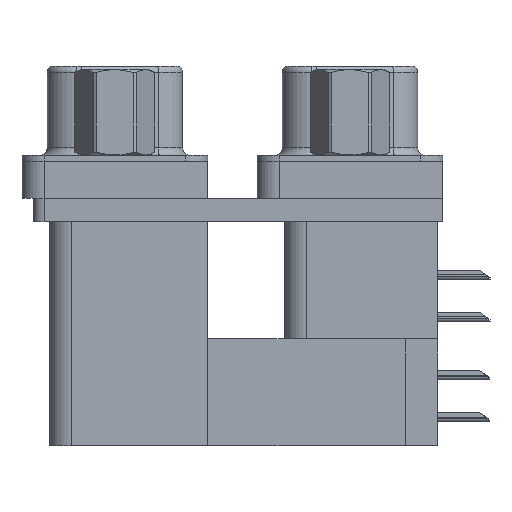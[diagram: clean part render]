
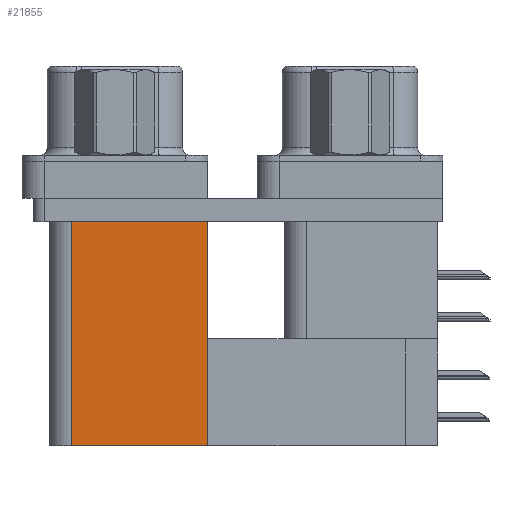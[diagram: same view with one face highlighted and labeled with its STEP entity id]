
A CAD part, left-side view. The second image highlights one B-rep face of the part: STEP entity #21855.
In plain terms, the highlighted planar face has unit normal (-1, 0, 0).
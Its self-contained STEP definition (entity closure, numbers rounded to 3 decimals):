
#1207 = PLANE ( 'NONE',  #14484 ) ;
#2067 = VERTEX_POINT ( 'NONE', #24775 ) ;
#2484 = VECTOR ( 'NONE', #4915, 1000. ) ;
#2681 = LINE ( 'NONE', #6771, #27761 ) ;
#4915 = DIRECTION ( 'NONE',  ( 0., 0., 1. ) ) ;
#5974 = VERTEX_POINT ( 'NONE', #7982 ) ;
#6165 = DIRECTION ( 'NONE',  ( 0., 0., 1. ) ) ;
#6771 = CARTESIAN_POINT ( 'NONE',  ( 3.7, 9.6, -19.2 ) ) ;
#7982 = CARTESIAN_POINT ( 'NONE',  ( 3.7, 9.6, -19.2 ) ) ;
#8665 = EDGE_CURVE ( 'NONE', #5974, #22039, #2681, .T. ) ;
#9884 = ORIENTED_EDGE ( 'NONE', *, *, #22819, .F. ) ;
#11655 = CARTESIAN_POINT ( 'NONE',  ( 3.7, 9.6, -19.2 ) ) ;
#13411 = LINE ( 'NONE', #20430, #40462 ) ;
#14484 = AXIS2_PLACEMENT_3D ( 'NONE', #11655, #32255, #31804 ) ;
#20430 = CARTESIAN_POINT ( 'NONE',  ( 3.7, 18.8, -19.2 ) ) ;
#20454 = CARTESIAN_POINT ( 'NONE',  ( 3.7, 18.8, -19.2 ) ) ;
#20587 = DIRECTION ( 'NONE',  ( 0., 1., 0. ) ) ;
#20968 = ORIENTED_EDGE ( 'NONE', *, *, #8665, .F. ) ;
#21855 = ADVANCED_FACE ( 'NONE', ( #35194 ), #1207, .F. ) ;
#22039 = VERTEX_POINT ( 'NONE', #20454 ) ;
#22819 = EDGE_CURVE ( 'NONE', #22039, #27255, #13411, .T. ) ;
#23968 = ORIENTED_EDGE ( 'NONE', *, *, #31634, .T. ) ;
#24775 = CARTESIAN_POINT ( 'NONE',  ( 3.7, 9.6, -2.5 ) ) ;
#26036 = DIRECTION ( 'NONE',  ( 0., 1., 0. ) ) ;
#26537 = CARTESIAN_POINT ( 'NONE',  ( 3.7, 18.8, -2.5 ) ) ;
#27255 = VERTEX_POINT ( 'NONE', #26537 ) ;
#27761 = VECTOR ( 'NONE', #20587, 1000. ) ;
#29147 = CARTESIAN_POINT ( 'NONE',  ( 3.7, 9.6, -19.2 ) ) ;
#31634 = EDGE_CURVE ( 'NONE', #2067, #27255, #36011, .T. ) ;
#31804 = DIRECTION ( 'NONE',  ( 0., 0., -1. ) ) ;
#32255 = DIRECTION ( 'NONE',  ( 1., 0., 0. ) ) ;
#32833 = CARTESIAN_POINT ( 'NONE',  ( 3.7, 9.6, -2.5 ) ) ;
#35194 = FACE_OUTER_BOUND ( 'NONE', #42204, .T. ) ;
#36011 = LINE ( 'NONE', #32833, #44172 ) ;
#36355 = EDGE_CURVE ( 'NONE', #5974, #2067, #43197, .T. ) ;
#40462 = VECTOR ( 'NONE', #6165, 1000. ) ;
#42204 = EDGE_LOOP ( 'NONE', ( #23968, #9884, #20968, #44137 ) ) ;
#43197 = LINE ( 'NONE', #29147, #2484 ) ;
#44137 = ORIENTED_EDGE ( 'NONE', *, *, #36355, .T. ) ;
#44172 = VECTOR ( 'NONE', #26036, 1000. ) ;
